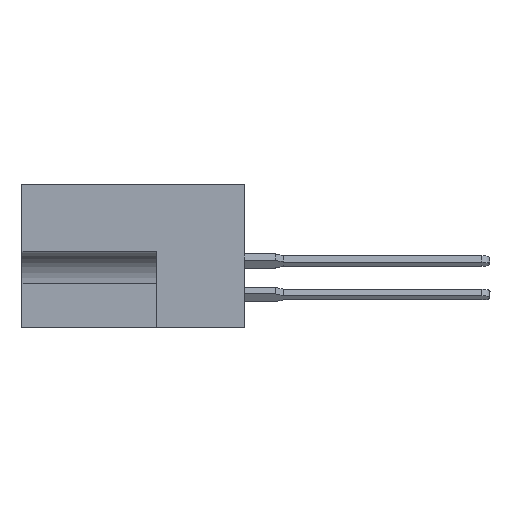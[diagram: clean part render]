
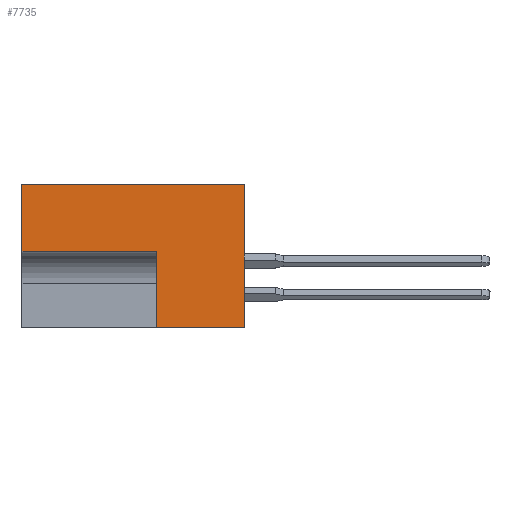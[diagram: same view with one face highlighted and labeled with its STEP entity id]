
A CAD part, left-side view. The second image highlights one B-rep face of the part: STEP entity #7735.
In plain terms, the highlighted planar face has unit normal (-1, 0, 0).
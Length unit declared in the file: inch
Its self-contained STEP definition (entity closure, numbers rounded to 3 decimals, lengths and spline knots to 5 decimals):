
#177 = DIRECTION ( 'NONE',  ( 0., -1., 0. ) ) ;
#460 = EDGE_CURVE ( 'NONE', #8222, #11520, #23232, .T. ) ;
#896 = EDGE_CURVE ( 'NONE', #11520, #25526, #16012, .T. ) ;
#1152 = DIRECTION ( 'NONE',  ( 0., 0., 1. ) ) ;
#1638 = CARTESIAN_POINT ( 'NONE',  ( 0., 0., -0.531 ) ) ;
#2447 = CARTESIAN_POINT ( 'NONE',  ( 0., 0.328, -0.248 ) ) ;
#4310 = EDGE_CURVE ( 'NONE', #23257, #8222, #9731, .T. ) ;
#4479 = VECTOR ( 'NONE', #1152, 39.37008 ) ;
#5740 = ORIENTED_EDGE ( 'NONE', *, *, #24000, .F. ) ;
#5916 = FACE_OUTER_BOUND ( 'NONE', #11800, .T. ) ;
#6081 = LINE ( 'NONE', #24615, #10984 ) ;
#6306 = DIRECTION ( 'NONE',  ( 1., 0., 0. ) ) ;
#7229 = ORIENTED_EDGE ( 'NONE', *, *, #896, .F. ) ;
#7735 = ADVANCED_FACE ( 'NONE', ( #5916 ), #8511, .F. ) ;
#8222 = VERTEX_POINT ( 'NONE', #19905 ) ;
#8358 = DIRECTION ( 'NONE',  ( 0., 1., 0. ) ) ;
#8511 = PLANE ( 'NONE',  #23095 ) ;
#8914 = CARTESIAN_POINT ( 'NONE',  ( 0., 0.328, -0.531 ) ) ;
#9380 = LINE ( 'NONE', #9421, #4479 ) ;
#9421 = CARTESIAN_POINT ( 'NONE',  ( 0., 0., 0. ) ) ;
#9731 = LINE ( 'NONE', #16954, #24067 ) ;
#9996 = EDGE_CURVE ( 'NONE', #16545, #12824, #9380, .T. ) ;
#10316 = EDGE_CURVE ( 'NONE', #23257, #16545, #6081, .T. ) ;
#10419 = DIRECTION ( 'NONE',  ( 0., 0., -1. ) ) ;
#10984 = VECTOR ( 'NONE', #18620, 39.37008 ) ;
#11170 = VECTOR ( 'NONE', #8358, 39.37008 ) ;
#11520 = VERTEX_POINT ( 'NONE', #20723 ) ;
#11800 = EDGE_LOOP ( 'NONE', ( #7229, #25715, #26609, #16117, #26818, #5740 ) ) ;
#12824 = VERTEX_POINT ( 'NONE', #21277 ) ;
#13981 = DIRECTION ( 'NONE',  ( 0., 0., 1. ) ) ;
#16012 = LINE ( 'NONE', #22288, #22879 ) ;
#16117 = ORIENTED_EDGE ( 'NONE', *, *, #10316, .T. ) ;
#16545 = VERTEX_POINT ( 'NONE', #1638 ) ;
#16751 = CARTESIAN_POINT ( 'NONE',  ( 0., 0.453, 0. ) ) ;
#16954 = CARTESIAN_POINT ( 'NONE',  ( 0., 0.328, -0.531 ) ) ;
#18272 = LINE ( 'NONE', #16751, #24467 ) ;
#18620 = DIRECTION ( 'NONE',  ( 0., -1., 0. ) ) ;
#19905 = CARTESIAN_POINT ( 'NONE',  ( 0., 0.328, -0.248 ) ) ;
#20697 = CARTESIAN_POINT ( 'NONE',  ( 0., 0.453, 0. ) ) ;
#20723 = CARTESIAN_POINT ( 'NONE',  ( 0., 0.828, -0.248 ) ) ;
#21277 = CARTESIAN_POINT ( 'NONE',  ( 0., 0., 0. ) ) ;
#21998 = CARTESIAN_POINT ( 'NONE',  ( 0., 0.828, 0. ) ) ;
#22288 = CARTESIAN_POINT ( 'NONE',  ( 0., 0.828, 0. ) ) ;
#22879 = VECTOR ( 'NONE', #13981, 39.37008 ) ;
#23001 = DIRECTION ( 'NONE',  ( 0., 0., 1. ) ) ;
#23095 = AXIS2_PLACEMENT_3D ( 'NONE', #20697, #6306, #10419 ) ;
#23232 = LINE ( 'NONE', #2447, #11170 ) ;
#23257 = VERTEX_POINT ( 'NONE', #8914 ) ;
#24000 = EDGE_CURVE ( 'NONE', #25526, #12824, #18272, .T. ) ;
#24067 = VECTOR ( 'NONE', #23001, 39.37008 ) ;
#24467 = VECTOR ( 'NONE', #177, 39.37008 ) ;
#24615 = CARTESIAN_POINT ( 'NONE',  ( 0., 0.453, -0.531 ) ) ;
#25526 = VERTEX_POINT ( 'NONE', #21998 ) ;
#25715 = ORIENTED_EDGE ( 'NONE', *, *, #460, .F. ) ;
#26609 = ORIENTED_EDGE ( 'NONE', *, *, #4310, .F. ) ;
#26818 = ORIENTED_EDGE ( 'NONE', *, *, #9996, .T. ) ;
